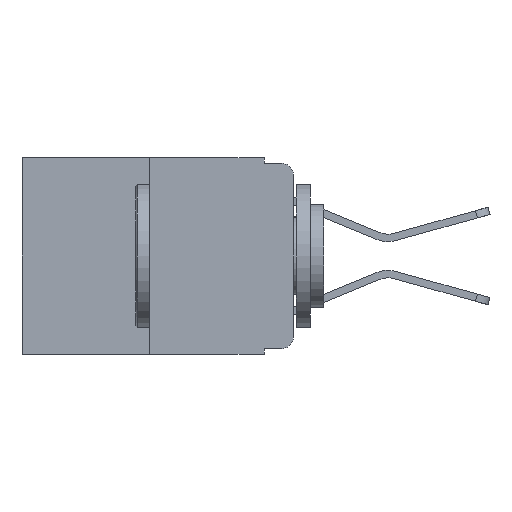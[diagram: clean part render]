
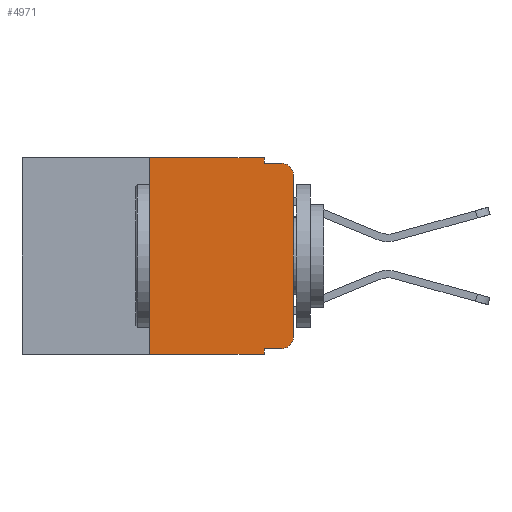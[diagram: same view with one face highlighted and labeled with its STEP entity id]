
A CAD part, left-side view. The second image highlights one B-rep face of the part: STEP entity #4971.
In plain terms, the highlighted planar face has unit normal (-1, 0, 0).
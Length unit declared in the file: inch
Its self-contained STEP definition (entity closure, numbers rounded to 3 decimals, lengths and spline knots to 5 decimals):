
#121 = CARTESIAN_POINT ( 'NONE',  ( 0., 0.02, -0.03 ) ) ;
#186 = DIRECTION ( 'NONE',  ( 0., 0., 1. ) ) ;
#240 = EDGE_LOOP ( 'NONE', ( #15196, #10712, #4753, #9949, #13087, #8886, #9017, #12150, #14562, #2817 ) ) ;
#252 = CARTESIAN_POINT ( 'NONE',  ( 0., 0.02, -0.313 ) ) ;
#480 = VERTEX_POINT ( 'NONE', #483 ) ;
#483 = CARTESIAN_POINT ( 'NONE',  ( 0., 0.051, -0.01 ) ) ;
#515 = LINE ( 'NONE', #12499, #4201 ) ;
#978 = VECTOR ( 'NONE', #13776, 39.37008 ) ;
#1017 = AXIS2_PLACEMENT_3D ( 'NONE', #13245, #6627, #13794 ) ;
#1079 = DIRECTION ( 'NONE',  ( 0., -1., 0. ) ) ;
#1382 = CARTESIAN_POINT ( 'NONE',  ( 0., 0.25, -0.343 ) ) ;
#1398 = VECTOR ( 'NONE', #5583, 39.37008 ) ;
#1552 = DIRECTION ( 'NONE',  ( 0., 0., -1. ) ) ;
#1675 = DIRECTION ( 'NONE',  ( 0., 0., -1. ) ) ;
#1843 = LINE ( 'NONE', #2903, #1398 ) ;
#2067 = VECTOR ( 'NONE', #1079, 39.37008 ) ;
#2817 = ORIENTED_EDGE ( 'NONE', *, *, #7692, .T. ) ;
#2903 = CARTESIAN_POINT ( 'NONE',  ( 0., 0., 0. ) ) ;
#2957 = DIRECTION ( 'NONE',  ( 0., 0., -1. ) ) ;
#4201 = VECTOR ( 'NONE', #5765, 39.37008 ) ;
#4261 = DIRECTION ( 'NONE',  ( 0., -1., 0. ) ) ;
#4636 = LINE ( 'NONE', #16343, #978 ) ;
#4753 = ORIENTED_EDGE ( 'NONE', *, *, #7641, .F. ) ;
#4971 = ADVANCED_FACE ( 'NONE', ( #13379 ), #6643, .F. ) ;
#5068 = CIRCLE ( 'NONE', #15013, 0.02 ) ;
#5583 = DIRECTION ( 'NONE',  ( 0., 0., 1. ) ) ;
#5603 = DIRECTION ( 'NONE',  ( 0., -1., 0. ) ) ;
#5765 = DIRECTION ( 'NONE',  ( 0., -1., 0. ) ) ;
#5800 = VERTEX_POINT ( 'NONE', #7631 ) ;
#6055 = VERTEX_POINT ( 'NONE', #7347 ) ;
#6627 = DIRECTION ( 'NONE',  ( 1., 0., 0. ) ) ;
#6643 = PLANE ( 'NONE',  #1017 ) ;
#7138 = EDGE_CURVE ( 'NONE', #6055, #14304, #12502, .T. ) ;
#7347 = CARTESIAN_POINT ( 'NONE',  ( 0., 0.25, 0. ) ) ;
#7376 = CIRCLE ( 'NONE', #16760, 0.02 ) ;
#7451 = EDGE_CURVE ( 'NONE', #15062, #8424, #12895, .T. ) ;
#7631 = CARTESIAN_POINT ( 'NONE',  ( 0., 0.02, -0.333 ) ) ;
#7635 = EDGE_CURVE ( 'NONE', #14649, #7911, #1843, .T. ) ;
#7638 = EDGE_CURVE ( 'NONE', #7911, #14708, #5068, .T. ) ;
#7641 = EDGE_CURVE ( 'NONE', #480, #14708, #8646, .T. ) ;
#7660 = EDGE_CURVE ( 'NONE', #14304, #480, #4636, .T. ) ;
#7665 = EDGE_CURVE ( 'NONE', #15062, #6055, #14957, .T. ) ;
#7687 = EDGE_CURVE ( 'NONE', #16238, #8424, #14560, .T. ) ;
#7690 = EDGE_CURVE ( 'NONE', #16238, #5800, #515, .T. ) ;
#7692 = EDGE_CURVE ( 'NONE', #5800, #14649, #7376, .T. ) ;
#7795 = VECTOR ( 'NONE', #186, 39.37008 ) ;
#7814 = CARTESIAN_POINT ( 'NONE',  ( 0., 0.473, -0.343 ) ) ;
#7911 = VERTEX_POINT ( 'NONE', #16970 ) ;
#8333 = CARTESIAN_POINT ( 'NONE',  ( 0., 0.051, -0.01 ) ) ;
#8393 = CARTESIAN_POINT ( 'NONE',  ( 0., 0.051, 0. ) ) ;
#8424 = VERTEX_POINT ( 'NONE', #15970 ) ;
#8611 = CARTESIAN_POINT ( 'NONE',  ( 0., 0.02, -0.01 ) ) ;
#8646 = LINE ( 'NONE', #8333, #11862 ) ;
#8886 = ORIENTED_EDGE ( 'NONE', *, *, #7665, .F. ) ;
#9017 = ORIENTED_EDGE ( 'NONE', *, *, #7451, .T. ) ;
#9427 = CARTESIAN_POINT ( 'NONE',  ( 0., 0.051, -0.333 ) ) ;
#9713 = DIRECTION ( 'NONE',  ( -1., 0., 0. ) ) ;
#9833 = DIRECTION ( 'NONE',  ( -1., 0., 0. ) ) ;
#9949 = ORIENTED_EDGE ( 'NONE', *, *, #7660, .F. ) ;
#10712 = ORIENTED_EDGE ( 'NONE', *, *, #7638, .T. ) ;
#10999 = VECTOR ( 'NONE', #2957, 39.37008 ) ;
#11188 = CARTESIAN_POINT ( 'NONE',  ( 0., 0., -0.313 ) ) ;
#11862 = VECTOR ( 'NONE', #4261, 39.37008 ) ;
#12150 = ORIENTED_EDGE ( 'NONE', *, *, #7687, .F. ) ;
#12499 = CARTESIAN_POINT ( 'NONE',  ( 0., 0.051, -0.333 ) ) ;
#12502 = LINE ( 'NONE', #16244, #15191 ) ;
#12895 = LINE ( 'NONE', #7814, #2067 ) ;
#13069 = CARTESIAN_POINT ( 'NONE',  ( 0., 0.051, 0. ) ) ;
#13087 = ORIENTED_EDGE ( 'NONE', *, *, #7138, .F. ) ;
#13245 = CARTESIAN_POINT ( 'NONE',  ( 0., 0.473, 0. ) ) ;
#13379 = FACE_OUTER_BOUND ( 'NONE', #240, .T. ) ;
#13776 = DIRECTION ( 'NONE',  ( 0., 0., -1. ) ) ;
#13794 = DIRECTION ( 'NONE',  ( 0., 0., -1. ) ) ;
#14304 = VERTEX_POINT ( 'NONE', #13069 ) ;
#14560 = LINE ( 'NONE', #8393, #10999 ) ;
#14562 = ORIENTED_EDGE ( 'NONE', *, *, #7690, .T. ) ;
#14649 = VERTEX_POINT ( 'NONE', #11188 ) ;
#14708 = VERTEX_POINT ( 'NONE', #8611 ) ;
#14957 = LINE ( 'NONE', #16400, #7795 ) ;
#15013 = AXIS2_PLACEMENT_3D ( 'NONE', #121, #9713, #1552 ) ;
#15062 = VERTEX_POINT ( 'NONE', #1382 ) ;
#15191 = VECTOR ( 'NONE', #5603, 39.37008 ) ;
#15196 = ORIENTED_EDGE ( 'NONE', *, *, #7635, .T. ) ;
#15970 = CARTESIAN_POINT ( 'NONE',  ( 0., 0.051, -0.343 ) ) ;
#16238 = VERTEX_POINT ( 'NONE', #9427 ) ;
#16244 = CARTESIAN_POINT ( 'NONE',  ( 0., 0.473, 0. ) ) ;
#16343 = CARTESIAN_POINT ( 'NONE',  ( 0., 0.051, 0. ) ) ;
#16400 = CARTESIAN_POINT ( 'NONE',  ( 0., 0.25, 0. ) ) ;
#16760 = AXIS2_PLACEMENT_3D ( 'NONE', #252, #9833, #1675 ) ;
#16970 = CARTESIAN_POINT ( 'NONE',  ( 0., 0., -0.03 ) ) ;
